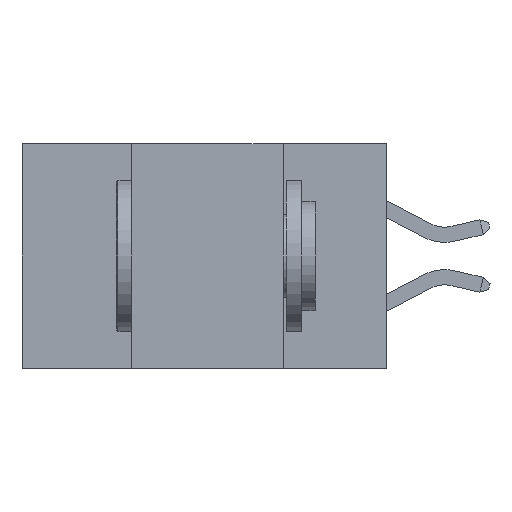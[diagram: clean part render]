
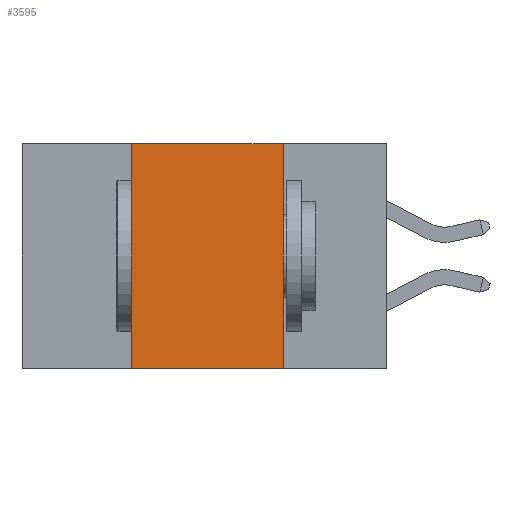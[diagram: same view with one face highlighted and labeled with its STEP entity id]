
A CAD part, left-side view. The second image highlights one B-rep face of the part: STEP entity #3595.
In plain terms, the highlighted planar face has unit normal (-1, 0, 0).
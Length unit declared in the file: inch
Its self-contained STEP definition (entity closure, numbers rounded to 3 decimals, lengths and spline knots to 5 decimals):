
#236 = CARTESIAN_POINT ( 'NONE',  ( 0., 0.17, -0.37 ) ) ;
#727 = VERTEX_POINT ( 'NONE', #236 ) ;
#2860 = DIRECTION ( 'NONE',  ( 1., 0., 0. ) ) ;
#3188 = DIRECTION ( 'NONE',  ( 0., 0., 1. ) ) ;
#3555 = CARTESIAN_POINT ( 'NONE',  ( 0., 0.6, -0.37 ) ) ;
#3595 = ADVANCED_FACE ( 'NONE', ( #16051 ), #24754, .F. ) ;
#3689 = DIRECTION ( 'NONE',  ( 0., -1., 0. ) ) ;
#4108 = LINE ( 'NONE', #17691, #24699 ) ;
#4217 = EDGE_CURVE ( 'NONE', #13048, #727, #18295, .T. ) ;
#4693 = AXIS2_PLACEMENT_3D ( 'NONE', #16524, #2860, #18536 ) ;
#4725 = EDGE_LOOP ( 'NONE', ( #6223, #18145, #5138, #5574 ) ) ;
#4754 = EDGE_CURVE ( 'NONE', #6496, #13048, #4108, .T. ) ;
#5138 = ORIENTED_EDGE ( 'NONE', *, *, #12393, .F. ) ;
#5574 = ORIENTED_EDGE ( 'NONE', *, *, #8483, .T. ) ;
#6223 = ORIENTED_EDGE ( 'NONE', *, *, #4217, .F. ) ;
#6231 = CARTESIAN_POINT ( 'NONE',  ( 0., 0.42, 0. ) ) ;
#6437 = CARTESIAN_POINT ( 'NONE',  ( 0., 0.17, 0. ) ) ;
#6496 = VERTEX_POINT ( 'NONE', #6231 ) ;
#8483 = EDGE_CURVE ( 'NONE', #19705, #727, #8549, .T. ) ;
#8549 = LINE ( 'NONE', #3555, #17245 ) ;
#12393 = EDGE_CURVE ( 'NONE', #19705, #6496, #22735, .T. ) ;
#13048 = VERTEX_POINT ( 'NONE', #18108 ) ;
#13186 = CARTESIAN_POINT ( 'NONE',  ( 0., 0.42, 0. ) ) ;
#13295 = DIRECTION ( 'NONE',  ( 0., -1., 0. ) ) ;
#16051 = FACE_OUTER_BOUND ( 'NONE', #4725, .T. ) ;
#16524 = CARTESIAN_POINT ( 'NONE',  ( 0., 0.6, 0. ) ) ;
#17245 = VECTOR ( 'NONE', #13295, 39.37008 ) ;
#17691 = CARTESIAN_POINT ( 'NONE',  ( 0., 0.6, 0. ) ) ;
#18000 = DIRECTION ( 'NONE',  ( 0., 0., -1. ) ) ;
#18108 = CARTESIAN_POINT ( 'NONE',  ( 0., 0.17, 0. ) ) ;
#18145 = ORIENTED_EDGE ( 'NONE', *, *, #4754, .F. ) ;
#18295 = LINE ( 'NONE', #6437, #23597 ) ;
#18536 = DIRECTION ( 'NONE',  ( 0., 0., -1. ) ) ;
#19705 = VERTEX_POINT ( 'NONE', #20138 ) ;
#20138 = CARTESIAN_POINT ( 'NONE',  ( 0., 0.42, -0.37 ) ) ;
#22735 = LINE ( 'NONE', #13186, #23723 ) ;
#23597 = VECTOR ( 'NONE', #18000, 39.37008 ) ;
#23723 = VECTOR ( 'NONE', #3188, 39.37008 ) ;
#24699 = VECTOR ( 'NONE', #3689, 39.37008 ) ;
#24754 = PLANE ( 'NONE',  #4693 ) ;
